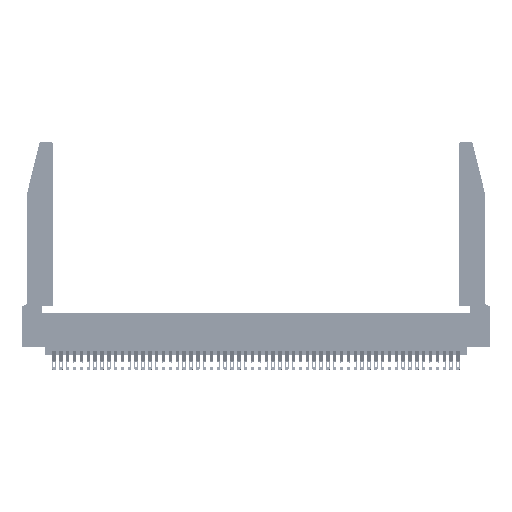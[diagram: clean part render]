
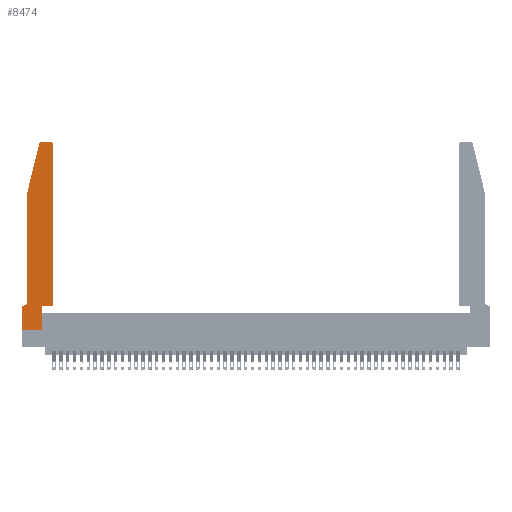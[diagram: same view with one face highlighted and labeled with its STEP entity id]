
A CAD part, top view. The second image highlights one B-rep face of the part: STEP entity #8474.
In plain terms, the highlighted planar face has unit normal (0, 0, 1).
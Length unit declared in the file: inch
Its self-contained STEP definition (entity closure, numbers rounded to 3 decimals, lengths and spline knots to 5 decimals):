
#85 = EDGE_CURVE ( 'NONE', #30790, #114, #39610, .T. ) ;
#114 = VERTEX_POINT ( 'NONE', #29039 ) ;
#536 = CARTESIAN_POINT ( 'NONE',  ( 0., 0., 0.37 ) ) ;
#1853 = CARTESIAN_POINT ( 'NONE',  ( 0.2605, 2.75, 0.37 ) ) ;
#2589 = CARTESIAN_POINT ( 'NONE',  ( 0.2865, 0., 0.37 ) ) ;
#3430 = CARTESIAN_POINT ( 'NONE',  ( 0.284, 2.72, 0.37 ) ) ;
#4059 = VERTEX_POINT ( 'NONE', #48460 ) ;
#4182 = AXIS2_PLACEMENT_3D ( 'NONE', #44535, #48441, #47935 ) ;
#4201 = VERTEX_POINT ( 'NONE', #49113 ) ;
#4347 = DIRECTION ( 'NONE',  ( 0., -1., 0. ) ) ;
#4350 = CIRCLE ( 'NONE', #13083, 0.03 ) ;
#5282 = AXIS2_PLACEMENT_3D ( 'NONE', #17241, #40676, #5453 ) ;
#5453 = DIRECTION ( 'NONE',  ( -1., 0., 0. ) ) ;
#6496 = VERTEX_POINT ( 'NONE', #19194 ) ;
#6732 = CARTESIAN_POINT ( 'NONE',  ( 0., 0., 0.37 ) ) ;
#6930 = ORIENTED_EDGE ( 'NONE', *, *, #40571, .T. ) ;
#6993 = EDGE_CURVE ( 'NONE', #114, #4059, #15592, .T. ) ;
#8289 = FACE_OUTER_BOUND ( 'NONE', #35029, .T. ) ;
#8474 = ADVANCED_FACE ( 'NONE', ( #8289 ), #9393, .T. ) ;
#8637 = EDGE_CURVE ( 'NONE', #4201, #6496, #18495, .T. ) ;
#8810 = ORIENTED_EDGE ( 'NONE', *, *, #13237, .T. ) ;
#9162 = EDGE_CURVE ( 'NONE', #47888, #41042, #33928, .T. ) ;
#9225 = DIRECTION ( 'NONE',  ( 1., 0., 0. ) ) ;
#9393 = PLANE ( 'NONE',  #33237 ) ;
#9715 = DIRECTION ( 'NONE',  ( 0., 1., 0. ) ) ;
#9922 = EDGE_CURVE ( 'NONE', #41042, #36820, #41391, .T. ) ;
#10874 = CARTESIAN_POINT ( 'NONE',  ( 0.0755, 2., 0.37 ) ) ;
#11141 = DIRECTION ( 'NONE',  ( 1., 0., 0. ) ) ;
#11618 = ORIENTED_EDGE ( 'NONE', *, *, #6993, .T. ) ;
#11652 = VECTOR ( 'NONE', #12136, 39.37008 ) ;
#12136 = DIRECTION ( 'NONE',  ( 0., -1., 0. ) ) ;
#12382 = LINE ( 'NONE', #43409, #44946 ) ;
#12965 = CARTESIAN_POINT ( 'NONE',  ( 0., 0.35, 0.37 ) ) ;
#13083 = AXIS2_PLACEMENT_3D ( 'NONE', #3430, #34248, #11141 ) ;
#13237 = EDGE_CURVE ( 'NONE', #29813, #47888, #44715, .T. ) ;
#14687 = CIRCLE ( 'NONE', #4182, 0.03 ) ;
#14774 = DIRECTION ( 'NONE',  ( -0.239, -0.971, 0. ) ) ;
#14798 = CARTESIAN_POINT ( 'NONE',  ( 0.4505, 2.72, 0.37 ) ) ;
#15053 = VECTOR ( 'NONE', #36519, 39.37008 ) ;
#15592 = LINE ( 'NONE', #19483, #25833 ) ;
#16129 = ORIENTED_EDGE ( 'NONE', *, *, #43894, .T. ) ;
#17241 = CARTESIAN_POINT ( 'NONE',  ( 0.0055, 0.42, 0.37 ) ) ;
#17263 = DIRECTION ( 'NONE',  ( 1., 0., 0. ) ) ;
#17548 = ORIENTED_EDGE ( 'NONE', *, *, #20362, .T. ) ;
#17920 = VECTOR ( 'NONE', #44115, 39.37008 ) ;
#18495 = LINE ( 'NONE', #1853, #17920 ) ;
#18685 = CARTESIAN_POINT ( 'NONE',  ( 0.2865, 0.35, 0.37 ) ) ;
#19194 = CARTESIAN_POINT ( 'NONE',  ( 0.284, 2.75, 0.37 ) ) ;
#19483 = CARTESIAN_POINT ( 'NONE',  ( 0.0755, 0.35, 0.37 ) ) ;
#20362 = EDGE_CURVE ( 'NONE', #30964, #30790, #12382, .T. ) ;
#21161 = CARTESIAN_POINT ( 'NONE',  ( 0.2865, 0.35, 0.37 ) ) ;
#21558 = CARTESIAN_POINT ( 'NONE',  ( 0.4505, 0.35, 0.37 ) ) ;
#21826 = EDGE_CURVE ( 'NONE', #4059, #29813, #29734, .T. ) ;
#22322 = ORIENTED_EDGE ( 'NONE', *, *, #8637, .T. ) ;
#22429 = EDGE_CURVE ( 'NONE', #36820, #27114, #30149, .T. ) ;
#23294 = CARTESIAN_POINT ( 'NONE',  ( 0.0755, 2., 0.37 ) ) ;
#24610 = ORIENTED_EDGE ( 'NONE', *, *, #9162, .T. ) ;
#24688 = CARTESIAN_POINT ( 'NONE',  ( 0.4505, 0.35, 0.37 ) ) ;
#25833 = VECTOR ( 'NONE', #38882, 39.37008 ) ;
#25934 = DIRECTION ( 'NONE',  ( 1., 0., 0. ) ) ;
#27114 = VERTEX_POINT ( 'NONE', #14798 ) ;
#29039 = CARTESIAN_POINT ( 'NONE',  ( 0.0055, 0.35, 0.37 ) ) ;
#29734 = LINE ( 'NONE', #536, #11652 ) ;
#29813 = VERTEX_POINT ( 'NONE', #34610 ) ;
#29825 = VECTOR ( 'NONE', #14774, 39.37008 ) ;
#30149 = LINE ( 'NONE', #24688, #15053 ) ;
#30790 = VERTEX_POINT ( 'NONE', #41217 ) ;
#30964 = VERTEX_POINT ( 'NONE', #23294 ) ;
#31990 = VERTEX_POINT ( 'NONE', #33170 ) ;
#32489 = DIRECTION ( 'NONE',  ( 0., 0., 1. ) ) ;
#32967 = VECTOR ( 'NONE', #17263, 39.37008 ) ;
#33170 = CARTESIAN_POINT ( 'NONE',  ( 0.25487, 2.72718, 0.37 ) ) ;
#33237 = AXIS2_PLACEMENT_3D ( 'NONE', #12965, #32489, #9225 ) ;
#33928 = LINE ( 'NONE', #21161, #45503 ) ;
#34248 = DIRECTION ( 'NONE',  ( 0., 0., 1. ) ) ;
#34610 = CARTESIAN_POINT ( 'NONE',  ( 0., 0., 0.37 ) ) ;
#34886 = ORIENTED_EDGE ( 'NONE', *, *, #22429, .T. ) ;
#35029 = EDGE_LOOP ( 'NONE', ( #22322, #6930, #35151, #17548, #41482, #11618, #48015, #8810, #24610, #49580, #34886, #16129 ) ) ;
#35151 = ORIENTED_EDGE ( 'NONE', *, *, #37666, .T. ) ;
#36519 = DIRECTION ( 'NONE',  ( 0., 1., 0. ) ) ;
#36664 = CARTESIAN_POINT ( 'NONE',  ( 0.4505, 0.35, 0.37 ) ) ;
#36820 = VERTEX_POINT ( 'NONE', #21558 ) ;
#37666 = EDGE_CURVE ( 'NONE', #31990, #30964, #40091, .T. ) ;
#38882 = DIRECTION ( 'NONE',  ( -1., 0., 0. ) ) ;
#39610 = CIRCLE ( 'NONE', #5282, 0.07 ) ;
#40091 = LINE ( 'NONE', #10874, #29825 ) ;
#40536 = VECTOR ( 'NONE', #25934, 39.37008 ) ;
#40571 = EDGE_CURVE ( 'NONE', #6496, #31990, #4350, .T. ) ;
#40676 = DIRECTION ( 'NONE',  ( 0., 0., -1. ) ) ;
#41042 = VERTEX_POINT ( 'NONE', #18685 ) ;
#41217 = CARTESIAN_POINT ( 'NONE',  ( 0.0755, 0.42, 0.37 ) ) ;
#41391 = LINE ( 'NONE', #36664, #32967 ) ;
#41482 = ORIENTED_EDGE ( 'NONE', *, *, #85, .T. ) ;
#43409 = CARTESIAN_POINT ( 'NONE',  ( 0.0755, 2., 0.37 ) ) ;
#43894 = EDGE_CURVE ( 'NONE', #27114, #4201, #14687, .T. ) ;
#44115 = DIRECTION ( 'NONE',  ( -1., 0., 0. ) ) ;
#44535 = CARTESIAN_POINT ( 'NONE',  ( 0.4205, 2.72, 0.37 ) ) ;
#44715 = LINE ( 'NONE', #6732, #40536 ) ;
#44946 = VECTOR ( 'NONE', #4347, 39.37008 ) ;
#45503 = VECTOR ( 'NONE', #9715, 39.37008 ) ;
#47888 = VERTEX_POINT ( 'NONE', #2589 ) ;
#47935 = DIRECTION ( 'NONE',  ( 1., 0., 0. ) ) ;
#48015 = ORIENTED_EDGE ( 'NONE', *, *, #21826, .T. ) ;
#48441 = DIRECTION ( 'NONE',  ( 0., 0., 1. ) ) ;
#48460 = CARTESIAN_POINT ( 'NONE',  ( 0., 0.35, 0.37 ) ) ;
#49113 = CARTESIAN_POINT ( 'NONE',  ( 0.4205, 2.75, 0.37 ) ) ;
#49580 = ORIENTED_EDGE ( 'NONE', *, *, #9922, .T. ) ;
